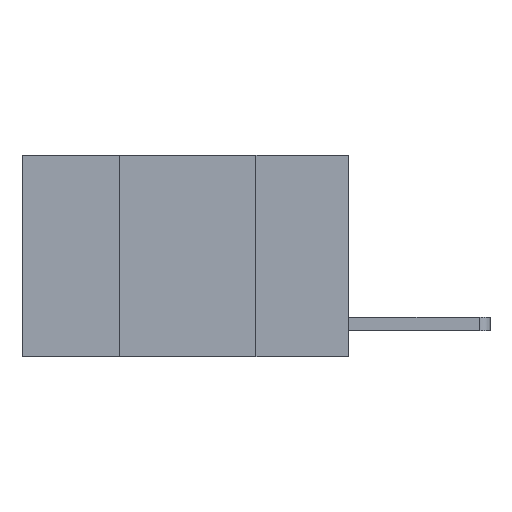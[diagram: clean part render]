
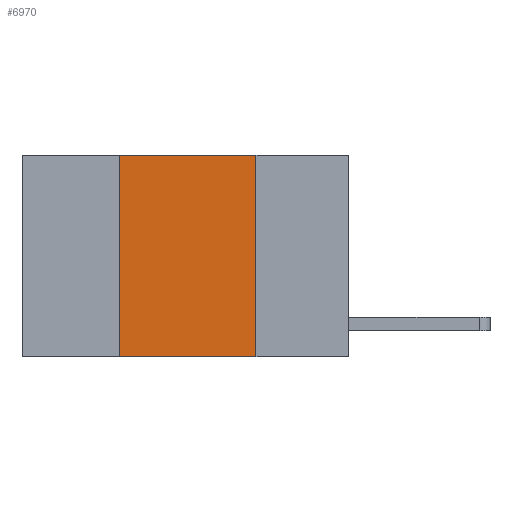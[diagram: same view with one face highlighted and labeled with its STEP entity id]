
A CAD part, left-side view. The second image highlights one B-rep face of the part: STEP entity #6970.
In plain terms, the highlighted planar face has unit normal (-1, 0, 0).
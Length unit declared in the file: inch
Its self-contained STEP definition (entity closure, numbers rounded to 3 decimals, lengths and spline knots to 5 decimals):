
#12 = PLANE ( 'NONE',  #4054 ) ;
#129 = VECTOR ( 'NONE', #2134, 39.37008 ) ;
#1171 = ORIENTED_EDGE ( 'NONE', *, *, #3333, .F. ) ;
#1223 = EDGE_CURVE ( 'NONE', #7636, #5992, #6650, .T. ) ;
#1305 = DIRECTION ( 'NONE',  ( 0., 0., -1. ) ) ;
#1387 = VECTOR ( 'NONE', #5920, 39.37008 ) ;
#1508 = CARTESIAN_POINT ( 'NONE',  ( 0., 0.6, -0.37 ) ) ;
#1566 = ORIENTED_EDGE ( 'NONE', *, *, #1223, .F. ) ;
#1719 = CARTESIAN_POINT ( 'NONE',  ( 0., 0.17, 0. ) ) ;
#1797 = DIRECTION ( 'NONE',  ( 0., 0., 1. ) ) ;
#1821 = CARTESIAN_POINT ( 'NONE',  ( 0., 0.42, 0. ) ) ;
#2029 = FACE_OUTER_BOUND ( 'NONE', #2961, .T. ) ;
#2134 = DIRECTION ( 'NONE',  ( 0., -1., 0. ) ) ;
#2355 = DIRECTION ( 'NONE',  ( 0., 0., -1. ) ) ;
#2743 = CARTESIAN_POINT ( 'NONE',  ( 0., 0.42, 0. ) ) ;
#2961 = EDGE_LOOP ( 'NONE', ( #1171, #5905, #1566, #7227 ) ) ;
#3073 = VERTEX_POINT ( 'NONE', #6462 ) ;
#3333 = EDGE_CURVE ( 'NONE', #6524, #3073, #3602, .T. ) ;
#3370 = CARTESIAN_POINT ( 'NONE',  ( 0., 0.42, -0.37 ) ) ;
#3513 = LINE ( 'NONE', #1508, #129 ) ;
#3602 = LINE ( 'NONE', #1719, #6275 ) ;
#4054 = AXIS2_PLACEMENT_3D ( 'NONE', #4433, #5050, #1305 ) ;
#4433 = CARTESIAN_POINT ( 'NONE',  ( 0., 0.6, 0. ) ) ;
#4523 = LINE ( 'NONE', #5301, #1387 ) ;
#4999 = VECTOR ( 'NONE', #1797, 39.37008 ) ;
#5050 = DIRECTION ( 'NONE',  ( 1., 0., 0. ) ) ;
#5301 = CARTESIAN_POINT ( 'NONE',  ( 0., 0.6, 0. ) ) ;
#5797 = CARTESIAN_POINT ( 'NONE',  ( 0., 0.17, 0. ) ) ;
#5905 = ORIENTED_EDGE ( 'NONE', *, *, #6111, .F. ) ;
#5920 = DIRECTION ( 'NONE',  ( 0., -1., 0. ) ) ;
#5992 = VERTEX_POINT ( 'NONE', #2743 ) ;
#6111 = EDGE_CURVE ( 'NONE', #5992, #6524, #4523, .T. ) ;
#6275 = VECTOR ( 'NONE', #2355, 39.37008 ) ;
#6462 = CARTESIAN_POINT ( 'NONE',  ( 0., 0.17, -0.37 ) ) ;
#6524 = VERTEX_POINT ( 'NONE', #5797 ) ;
#6650 = LINE ( 'NONE', #1821, #4999 ) ;
#6970 = ADVANCED_FACE ( 'NONE', ( #2029 ), #12, .F. ) ;
#7227 = ORIENTED_EDGE ( 'NONE', *, *, #7663, .T. ) ;
#7636 = VERTEX_POINT ( 'NONE', #3370 ) ;
#7663 = EDGE_CURVE ( 'NONE', #7636, #3073, #3513, .T. ) ;
